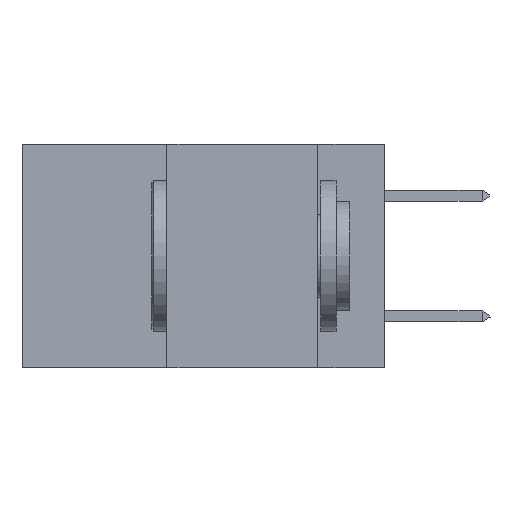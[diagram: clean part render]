
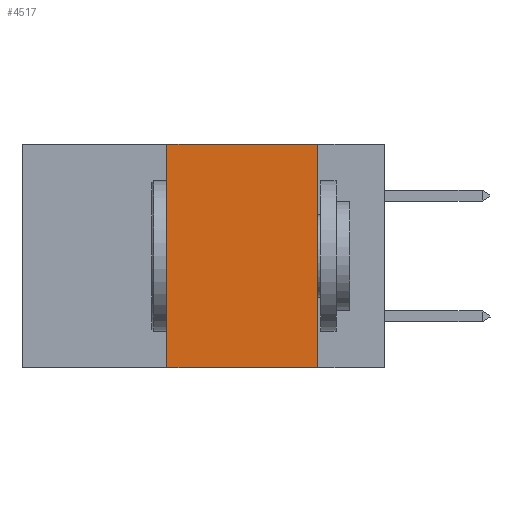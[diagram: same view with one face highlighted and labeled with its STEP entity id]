
A CAD part, left-side view. The second image highlights one B-rep face of the part: STEP entity #4517.
In plain terms, the highlighted planar face has unit normal (-1, 0, 0).
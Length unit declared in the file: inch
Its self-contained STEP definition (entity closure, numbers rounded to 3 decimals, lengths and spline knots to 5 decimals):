
#2800 = CARTESIAN_POINT ( 'NONE',  ( 0., 0.6, 0. ) ) ;
#3312 = CARTESIAN_POINT ( 'NONE',  ( 0., 0.36, -0.37 ) ) ;
#4517 = ADVANCED_FACE ( 'NONE', ( #11812 ), #4982, .F. ) ;
#4878 = DIRECTION ( 'NONE',  ( 1., 0., 0. ) ) ;
#4982 = PLANE ( 'NONE',  #16141 ) ;
#6790 = VECTOR ( 'NONE', #12690, 39.37008 ) ;
#7010 = EDGE_CURVE ( 'NONE', #9381, #10498, #26171, .T. ) ;
#7145 = VERTEX_POINT ( 'NONE', #16555 ) ;
#8045 = VECTOR ( 'NONE', #26020, 39.37008 ) ;
#9318 = VERTEX_POINT ( 'NONE', #26519 ) ;
#9381 = VERTEX_POINT ( 'NONE', #3312 ) ;
#9798 = CARTESIAN_POINT ( 'NONE',  ( 0., 0.36, 0. ) ) ;
#10498 = VERTEX_POINT ( 'NONE', #20823 ) ;
#11812 = FACE_OUTER_BOUND ( 'NONE', #27817, .T. ) ;
#12374 = VECTOR ( 'NONE', #18141, 39.37008 ) ;
#12690 = DIRECTION ( 'NONE',  ( 0., 0., -1. ) ) ;
#12754 = CARTESIAN_POINT ( 'NONE',  ( 0., 0.6, -0.37 ) ) ;
#14576 = ORIENTED_EDGE ( 'NONE', *, *, #25358, .F. ) ;
#14646 = DIRECTION ( 'NONE',  ( 0., -1., 0. ) ) ;
#15427 = ORIENTED_EDGE ( 'NONE', *, *, #20515, .T. ) ;
#15711 = ORIENTED_EDGE ( 'NONE', *, *, #7010, .F. ) ;
#16141 = AXIS2_PLACEMENT_3D ( 'NONE', #2800, #4878, #26479 ) ;
#16555 = CARTESIAN_POINT ( 'NONE',  ( 0., 0.11, -0.37 ) ) ;
#18141 = DIRECTION ( 'NONE',  ( 0., 0., 1. ) ) ;
#18445 = ORIENTED_EDGE ( 'NONE', *, *, #27605, .F. ) ;
#20515 = EDGE_CURVE ( 'NONE', #9381, #7145, #22157, .T. ) ;
#20823 = CARTESIAN_POINT ( 'NONE',  ( 0., 0.36, 0. ) ) ;
#21361 = LINE ( 'NONE', #27665, #26102 ) ;
#22157 = LINE ( 'NONE', #12754, #8045 ) ;
#24652 = LINE ( 'NONE', #25591, #6790 ) ;
#25358 = EDGE_CURVE ( 'NONE', #10498, #9318, #21361, .T. ) ;
#25591 = CARTESIAN_POINT ( 'NONE',  ( 0., 0.11, 0. ) ) ;
#26020 = DIRECTION ( 'NONE',  ( 0., -1., 0. ) ) ;
#26102 = VECTOR ( 'NONE', #14646, 39.37008 ) ;
#26171 = LINE ( 'NONE', #9798, #12374 ) ;
#26479 = DIRECTION ( 'NONE',  ( 0., 0., -1. ) ) ;
#26519 = CARTESIAN_POINT ( 'NONE',  ( 0., 0.11, 0. ) ) ;
#27605 = EDGE_CURVE ( 'NONE', #9318, #7145, #24652, .T. ) ;
#27665 = CARTESIAN_POINT ( 'NONE',  ( 0., 0.6, 0. ) ) ;
#27817 = EDGE_LOOP ( 'NONE', ( #18445, #14576, #15711, #15427 ) ) ;
